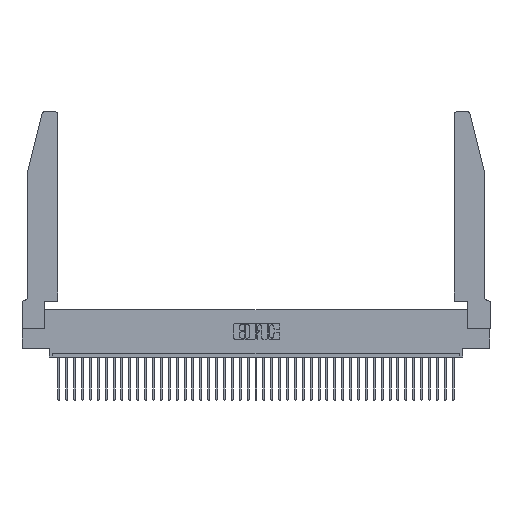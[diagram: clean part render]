
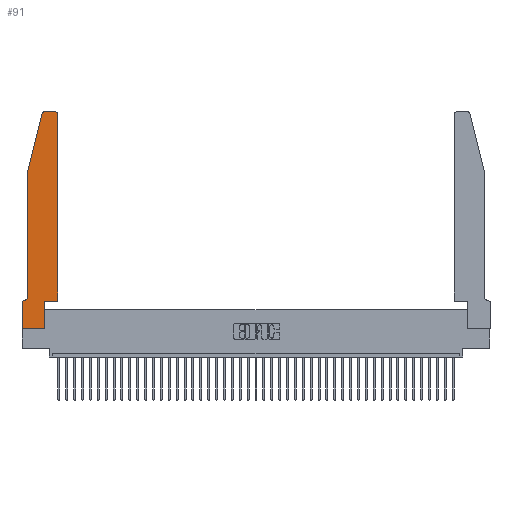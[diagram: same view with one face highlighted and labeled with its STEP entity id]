
A CAD part, top view. The second image highlights one B-rep face of the part: STEP entity #91.
In plain terms, the highlighted planar face has unit normal (0, 0, 1).
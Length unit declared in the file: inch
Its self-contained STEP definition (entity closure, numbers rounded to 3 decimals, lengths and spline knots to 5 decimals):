
#91 = ADVANCED_FACE ( 'NONE', ( #9376 ), #21477, .T. ) ;
#416 = VECTOR ( 'NONE', #33736, 39.37008 ) ;
#437 = DIRECTION ( 'NONE',  ( -1., 0., 0. ) ) ;
#490 = DIRECTION ( 'NONE',  ( 0., 0., 1. ) ) ;
#1461 = EDGE_CURVE ( 'NONE', #37072, #2426, #5141, .T. ) ;
#1626 = CARTESIAN_POINT ( 'NONE',  ( 0.25487, 2.72718, 0.37 ) ) ;
#1912 = DIRECTION ( 'NONE',  ( 1., 0., 0. ) ) ;
#2297 = VECTOR ( 'NONE', #14303, 39.37008 ) ;
#2300 = EDGE_CURVE ( 'NONE', #11489, #6519, #13149, .T. ) ;
#2366 = CARTESIAN_POINT ( 'NONE',  ( 0.2605, 2.75, 0.37 ) ) ;
#2426 = VERTEX_POINT ( 'NONE', #33242 ) ;
#2568 = ORIENTED_EDGE ( 'NONE', *, *, #9095, .T. ) ;
#3470 = ORIENTED_EDGE ( 'NONE', *, *, #1461, .T. ) ;
#4261 = ORIENTED_EDGE ( 'NONE', *, *, #37011, .T. ) ;
#4476 = ORIENTED_EDGE ( 'NONE', *, *, #20732, .T. ) ;
#4645 = CARTESIAN_POINT ( 'NONE',  ( 0.4505, 0.35, 0.37 ) ) ;
#5141 = LINE ( 'NONE', #8575, #21371 ) ;
#5335 = VERTEX_POINT ( 'NONE', #1626 ) ;
#5455 = ORIENTED_EDGE ( 'NONE', *, *, #23687, .T. ) ;
#5473 = CARTESIAN_POINT ( 'NONE',  ( 0.2865, 0.35, 0.37 ) ) ;
#5558 = CARTESIAN_POINT ( 'NONE',  ( 0.4505, 2.72, 0.37 ) ) ;
#5929 = VECTOR ( 'NONE', #32537, 39.37008 ) ;
#6519 = VERTEX_POINT ( 'NONE', #25108 ) ;
#6796 = CARTESIAN_POINT ( 'NONE',  ( 0.284, 2.72, 0.37 ) ) ;
#7879 = VERTEX_POINT ( 'NONE', #32135 ) ;
#8043 = AXIS2_PLACEMENT_3D ( 'NONE', #29934, #10997, #20460 ) ;
#8432 = DIRECTION ( 'NONE',  ( 0., -1., 0. ) ) ;
#8575 = CARTESIAN_POINT ( 'NONE',  ( 0., 0., 0.37 ) ) ;
#9095 = EDGE_CURVE ( 'NONE', #29883, #23485, #17593, .T. ) ;
#9376 = FACE_OUTER_BOUND ( 'NONE', #17755, .T. ) ;
#9476 = LINE ( 'NONE', #21177, #25204 ) ;
#10997 = DIRECTION ( 'NONE',  ( 0., 0., 1. ) ) ;
#11034 = CARTESIAN_POINT ( 'NONE',  ( 0.0755, 2., 0.37 ) ) ;
#11489 = VERTEX_POINT ( 'NONE', #27096 ) ;
#11564 = DIRECTION ( 'NONE',  ( 0., 0., 1. ) ) ;
#11568 = CARTESIAN_POINT ( 'NONE',  ( 0., 0.35, 0.37 ) ) ;
#11856 = CARTESIAN_POINT ( 'NONE',  ( 0., 0.35, 0.37 ) ) ;
#13114 = LINE ( 'NONE', #24890, #18225 ) ;
#13149 = CIRCLE ( 'NONE', #22690, 0.07 ) ;
#14303 = DIRECTION ( 'NONE',  ( 1., 0., 0. ) ) ;
#14471 = CARTESIAN_POINT ( 'NONE',  ( 0., 0., 0.37 ) ) ;
#14768 = DIRECTION ( 'NONE',  ( 0., 1., 0. ) ) ;
#14890 = VECTOR ( 'NONE', #27612, 39.37008 ) ;
#15439 = DIRECTION ( 'NONE',  ( -1., 0., 0. ) ) ;
#15710 = VERTEX_POINT ( 'NONE', #5558 ) ;
#16554 = VECTOR ( 'NONE', #15439, 39.37008 ) ;
#17593 = LINE ( 'NONE', #2366, #16554 ) ;
#17746 = LINE ( 'NONE', #14471, #416 ) ;
#17755 = EDGE_LOOP ( 'NONE', ( #2568, #41788, #5455, #4261, #23010, #4476, #3470, #23026, #40347, #27476, #22139, #23827 ) ) ;
#18225 = VECTOR ( 'NONE', #20903, 39.37008 ) ;
#19220 = AXIS2_PLACEMENT_3D ( 'NONE', #6796, #490, #36137 ) ;
#19483 = VERTEX_POINT ( 'NONE', #21341 ) ;
#20460 = DIRECTION ( 'NONE',  ( 1., 0., 0. ) ) ;
#20732 = EDGE_CURVE ( 'NONE', #6519, #37072, #13114, .T. ) ;
#20903 = DIRECTION ( 'NONE',  ( -1., 0., 0. ) ) ;
#21177 = CARTESIAN_POINT ( 'NONE',  ( 0.0755, 2., 0.37 ) ) ;
#21341 = CARTESIAN_POINT ( 'NONE',  ( 0.2865, 0., 0.37 ) ) ;
#21371 = VECTOR ( 'NONE', #8432, 39.37008 ) ;
#21477 = PLANE ( 'NONE',  #41954 ) ;
#22139 = ORIENTED_EDGE ( 'NONE', *, *, #22505, .T. ) ;
#22505 = EDGE_CURVE ( 'NONE', #7879, #15710, #36822, .T. ) ;
#22690 = AXIS2_PLACEMENT_3D ( 'NONE', #38615, #25676, #437 ) ;
#23010 = ORIENTED_EDGE ( 'NONE', *, *, #2300, .T. ) ;
#23026 = ORIENTED_EDGE ( 'NONE', *, *, #34811, .T. ) ;
#23485 = VERTEX_POINT ( 'NONE', #25406 ) ;
#23687 = EDGE_CURVE ( 'NONE', #5335, #29393, #24502, .T. ) ;
#23827 = ORIENTED_EDGE ( 'NONE', *, *, #23939, .T. ) ;
#23939 = EDGE_CURVE ( 'NONE', #15710, #29883, #36116, .T. ) ;
#24299 = EDGE_CURVE ( 'NONE', #23485, #5335, #31575, .T. ) ;
#24502 = LINE ( 'NONE', #37293, #14890 ) ;
#24890 = CARTESIAN_POINT ( 'NONE',  ( 0.0755, 0.35, 0.37 ) ) ;
#24963 = VERTEX_POINT ( 'NONE', #5473 ) ;
#25108 = CARTESIAN_POINT ( 'NONE',  ( 0.0055, 0.35, 0.37 ) ) ;
#25204 = VECTOR ( 'NONE', #30371, 39.37008 ) ;
#25406 = CARTESIAN_POINT ( 'NONE',  ( 0.284, 2.75, 0.37 ) ) ;
#25676 = DIRECTION ( 'NONE',  ( 0., 0., -1. ) ) ;
#26937 = CARTESIAN_POINT ( 'NONE',  ( 0.4205, 2.75, 0.37 ) ) ;
#27096 = CARTESIAN_POINT ( 'NONE',  ( 0.0755, 0.42, 0.37 ) ) ;
#27476 = ORIENTED_EDGE ( 'NONE', *, *, #29381, .T. ) ;
#27612 = DIRECTION ( 'NONE',  ( -0.239, -0.971, 0. ) ) ;
#27943 = EDGE_CURVE ( 'NONE', #19483, #24963, #34391, .T. ) ;
#28183 = LINE ( 'NONE', #4645, #2297 ) ;
#29381 = EDGE_CURVE ( 'NONE', #24963, #7879, #28183, .T. ) ;
#29393 = VERTEX_POINT ( 'NONE', #11034 ) ;
#29883 = VERTEX_POINT ( 'NONE', #26937 ) ;
#29934 = CARTESIAN_POINT ( 'NONE',  ( 0.4205, 2.72, 0.37 ) ) ;
#30371 = DIRECTION ( 'NONE',  ( 0., -1., 0. ) ) ;
#31575 = CIRCLE ( 'NONE', #19220, 0.03 ) ;
#32135 = CARTESIAN_POINT ( 'NONE',  ( 0.4505, 0.35, 0.37 ) ) ;
#32537 = DIRECTION ( 'NONE',  ( 0., 1., 0. ) ) ;
#33242 = CARTESIAN_POINT ( 'NONE',  ( 0., 0., 0.37 ) ) ;
#33309 = VECTOR ( 'NONE', #14768, 39.37008 ) ;
#33736 = DIRECTION ( 'NONE',  ( 1., 0., 0. ) ) ;
#34321 = CARTESIAN_POINT ( 'NONE',  ( 0.2865, 0.35, 0.37 ) ) ;
#34391 = LINE ( 'NONE', #34321, #33309 ) ;
#34811 = EDGE_CURVE ( 'NONE', #2426, #19483, #17746, .T. ) ;
#36116 = CIRCLE ( 'NONE', #8043, 0.03 ) ;
#36137 = DIRECTION ( 'NONE',  ( 1., 0., 0. ) ) ;
#36822 = LINE ( 'NONE', #39553, #5929 ) ;
#37011 = EDGE_CURVE ( 'NONE', #29393, #11489, #9476, .T. ) ;
#37072 = VERTEX_POINT ( 'NONE', #11568 ) ;
#37293 = CARTESIAN_POINT ( 'NONE',  ( 0.0755, 2., 0.37 ) ) ;
#38615 = CARTESIAN_POINT ( 'NONE',  ( 0.0055, 0.42, 0.37 ) ) ;
#39553 = CARTESIAN_POINT ( 'NONE',  ( 0.4505, 0.35, 0.37 ) ) ;
#40347 = ORIENTED_EDGE ( 'NONE', *, *, #27943, .T. ) ;
#41788 = ORIENTED_EDGE ( 'NONE', *, *, #24299, .T. ) ;
#41954 = AXIS2_PLACEMENT_3D ( 'NONE', #11856, #11564, #1912 ) ;
